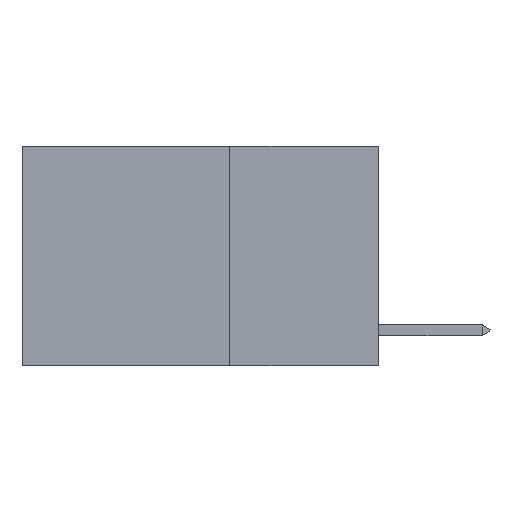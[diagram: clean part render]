
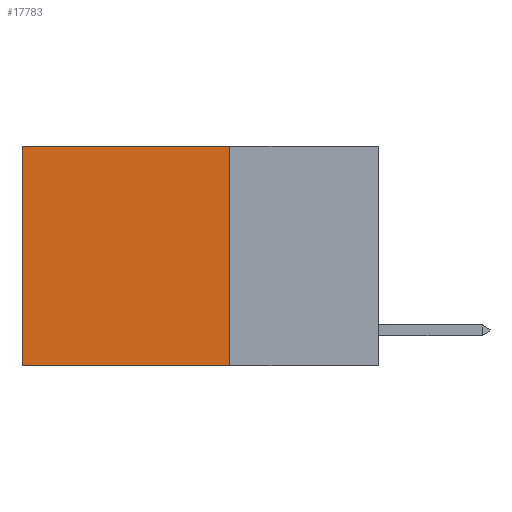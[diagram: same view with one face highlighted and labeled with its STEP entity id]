
A CAD part, left-side view. The second image highlights one B-rep face of the part: STEP entity #17783.
In plain terms, the highlighted planar face has unit normal (-1, 0, 0).
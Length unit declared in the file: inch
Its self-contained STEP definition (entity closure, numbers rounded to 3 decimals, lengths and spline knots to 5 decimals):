
#1648 = EDGE_CURVE ( 'NONE', #17861, #17533, #8700, .T. ) ;
#3325 = LINE ( 'NONE', #22787, #8585 ) ;
#3617 = ORIENTED_EDGE ( 'NONE', *, *, #1648, .T. ) ;
#4182 = DIRECTION ( 'NONE',  ( 1., 0., 0. ) ) ;
#4790 = VECTOR ( 'NONE', #22661, 39.37008 ) ;
#5171 = CARTESIAN_POINT ( 'NONE',  ( 0.2625, 0.25, 0. ) ) ;
#5568 = AXIS2_PLACEMENT_3D ( 'NONE', #5593, #4182, #9320 ) ;
#5593 = CARTESIAN_POINT ( 'NONE',  ( 0.2625, 0.25, 0. ) ) ;
#6144 = CARTESIAN_POINT ( 'NONE',  ( 0.2625, 0.25, 0. ) ) ;
#6589 = VERTEX_POINT ( 'NONE', #23128 ) ;
#6807 = LINE ( 'NONE', #5171, #21210 ) ;
#6829 = DIRECTION ( 'NONE',  ( 0., 0., -1. ) ) ;
#7050 = DIRECTION ( 'NONE',  ( 0., 1., 0. ) ) ;
#8120 = VERTEX_POINT ( 'NONE', #13047 ) ;
#8585 = VECTOR ( 'NONE', #6829, 39.37008 ) ;
#8700 = LINE ( 'NONE', #10446, #4790 ) ;
#9320 = DIRECTION ( 'NONE',  ( 0., 0., -1. ) ) ;
#9403 = ORIENTED_EDGE ( 'NONE', *, *, #22288, .T. ) ;
#10446 = CARTESIAN_POINT ( 'NONE',  ( 0.2625, 0.25, 0. ) ) ;
#10788 = EDGE_CURVE ( 'NONE', #17861, #6589, #6807, .T. ) ;
#10894 = LINE ( 'NONE', #12310, #13773 ) ;
#12310 = CARTESIAN_POINT ( 'NONE',  ( 0.2625, 0.25, -0.37 ) ) ;
#12340 = ORIENTED_EDGE ( 'NONE', *, *, #16788, .F. ) ;
#13047 = CARTESIAN_POINT ( 'NONE',  ( 0.2625, 0.6, -0.37 ) ) ;
#13773 = VECTOR ( 'NONE', #7050, 39.37008 ) ;
#15856 = EDGE_LOOP ( 'NONE', ( #9403, #12340, #21344, #3617 ) ) ;
#16788 = EDGE_CURVE ( 'NONE', #6589, #8120, #10894, .T. ) ;
#17456 = CARTESIAN_POINT ( 'NONE',  ( 0.2625, 0.6, 0. ) ) ;
#17533 = VERTEX_POINT ( 'NONE', #17456 ) ;
#17783 = ADVANCED_FACE ( 'NONE', ( #20013 ), #18242, .F. ) ;
#17861 = VERTEX_POINT ( 'NONE', #6144 ) ;
#18242 = PLANE ( 'NONE',  #5568 ) ;
#20013 = FACE_OUTER_BOUND ( 'NONE', #15856, .T. ) ;
#21125 = DIRECTION ( 'NONE',  ( 0., 0., -1. ) ) ;
#21210 = VECTOR ( 'NONE', #21125, 39.37008 ) ;
#21344 = ORIENTED_EDGE ( 'NONE', *, *, #10788, .F. ) ;
#22288 = EDGE_CURVE ( 'NONE', #17533, #8120, #3325, .T. ) ;
#22661 = DIRECTION ( 'NONE',  ( 0., 1., 0. ) ) ;
#22787 = CARTESIAN_POINT ( 'NONE',  ( 0.2625, 0.6, 0. ) ) ;
#23128 = CARTESIAN_POINT ( 'NONE',  ( 0.2625, 0.25, -0.37 ) ) ;
